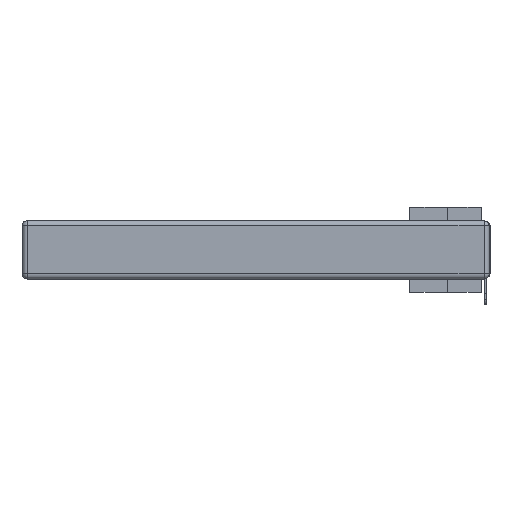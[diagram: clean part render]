
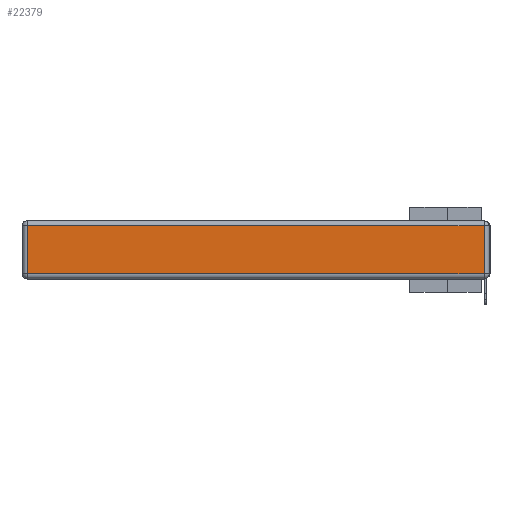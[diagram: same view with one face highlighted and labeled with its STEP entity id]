
A CAD part, left-side view. The second image highlights one B-rep face of the part: STEP entity #22379.
In plain terms, the highlighted planar face has unit normal (-1, 0, 0).
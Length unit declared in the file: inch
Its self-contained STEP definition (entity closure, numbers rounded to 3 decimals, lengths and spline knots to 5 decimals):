
#522 = CARTESIAN_POINT ( 'NONE',  ( 0., 2.72, -0.03 ) ) ;
#1147 = LINE ( 'NONE', #25175, #26015 ) ;
#1999 = VERTEX_POINT ( 'NONE', #33238 ) ;
#2948 = EDGE_CURVE ( 'NONE', #35361, #1999, #3924, .T. ) ;
#3924 = LINE ( 'NONE', #29486, #15510 ) ;
#5204 = EDGE_CURVE ( 'NONE', #35108, #35361, #10246, .T. ) ;
#6965 = CARTESIAN_POINT ( 'NONE',  ( 0., 0.03, -0.343 ) ) ;
#8780 = DIRECTION ( 'NONE',  ( 0., 0., 1. ) ) ;
#10095 = AXIS2_PLACEMENT_3D ( 'NONE', #29017, #20636, #8780 ) ;
#10246 = LINE ( 'NONE', #33563, #28459 ) ;
#10350 = EDGE_LOOP ( 'NONE', ( #25322, #23770, #29176, #10686 ) ) ;
#10686 = ORIENTED_EDGE ( 'NONE', *, *, #2948, .T. ) ;
#13984 = DIRECTION ( 'NONE',  ( 0., 0., -1. ) ) ;
#14451 = EDGE_CURVE ( 'NONE', #19433, #35108, #21077, .T. ) ;
#15510 = VECTOR ( 'NONE', #13984, 39.37008 ) ;
#15525 = FACE_OUTER_BOUND ( 'NONE', #10350, .T. ) ;
#19433 = VERTEX_POINT ( 'NONE', #31216 ) ;
#20636 = DIRECTION ( 'NONE',  ( -1., 0., 0. ) ) ;
#21077 = LINE ( 'NONE', #6965, #30777 ) ;
#22379 = ADVANCED_FACE ( 'NONE', ( #15525 ), #34603, .T. ) ;
#22594 = DIRECTION ( 'NONE',  ( 0., -1., 0. ) ) ;
#23770 = ORIENTED_EDGE ( 'NONE', *, *, #14451, .T. ) ;
#25175 = CARTESIAN_POINT ( 'NONE',  ( 0., 0., -0.313 ) ) ;
#25204 = EDGE_CURVE ( 'NONE', #1999, #19433, #1147, .T. ) ;
#25322 = ORIENTED_EDGE ( 'NONE', *, *, #25204, .T. ) ;
#26015 = VECTOR ( 'NONE', #22594, 39.37008 ) ;
#28459 = VECTOR ( 'NONE', #33333, 39.37008 ) ;
#29017 = CARTESIAN_POINT ( 'NONE',  ( 0., 0., -0.343 ) ) ;
#29176 = ORIENTED_EDGE ( 'NONE', *, *, #5204, .T. ) ;
#29486 = CARTESIAN_POINT ( 'NONE',  ( 0., 2.72, -0.343 ) ) ;
#30196 = CARTESIAN_POINT ( 'NONE',  ( 0., 0.03, -0.03 ) ) ;
#30777 = VECTOR ( 'NONE', #35399, 39.37008 ) ;
#31216 = CARTESIAN_POINT ( 'NONE',  ( 0., 0.03, -0.313 ) ) ;
#33238 = CARTESIAN_POINT ( 'NONE',  ( 0., 2.72, -0.313 ) ) ;
#33333 = DIRECTION ( 'NONE',  ( 0., 1., 0. ) ) ;
#33563 = CARTESIAN_POINT ( 'NONE',  ( 0., 2.75, -0.03 ) ) ;
#34603 = PLANE ( 'NONE',  #10095 ) ;
#35108 = VERTEX_POINT ( 'NONE', #30196 ) ;
#35361 = VERTEX_POINT ( 'NONE', #522 ) ;
#35399 = DIRECTION ( 'NONE',  ( 0., 0., 1. ) ) ;
